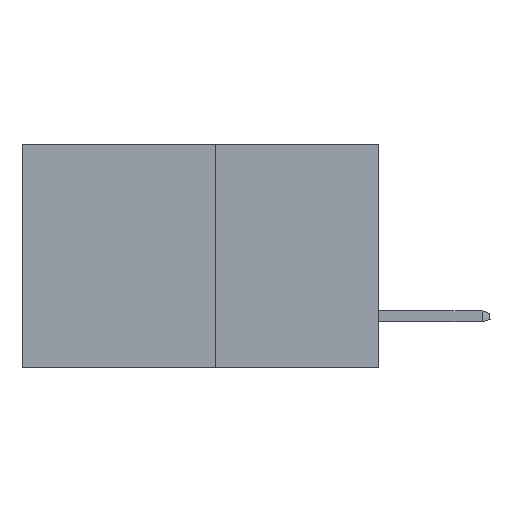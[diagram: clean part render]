
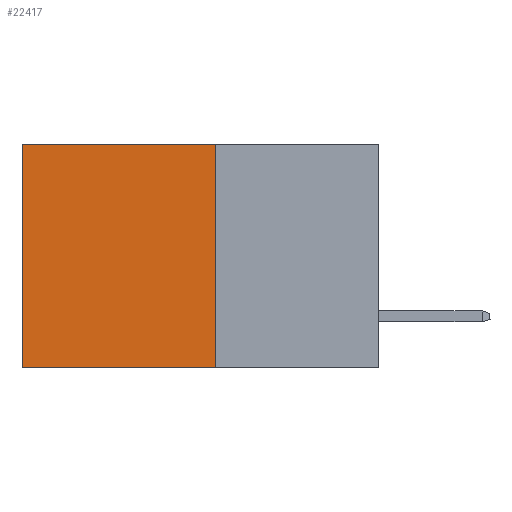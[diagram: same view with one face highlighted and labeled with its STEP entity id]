
A CAD part, left-side view. The second image highlights one B-rep face of the part: STEP entity #22417.
In plain terms, the highlighted planar face has unit normal (-1, 0, 0).
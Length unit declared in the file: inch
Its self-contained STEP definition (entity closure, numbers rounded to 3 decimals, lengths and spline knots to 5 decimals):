
#172 = VECTOR ( 'NONE', #13399, 39.37008 ) ;
#201 = LINE ( 'NONE', #4237, #14209 ) ;
#936 = VERTEX_POINT ( 'NONE', #5504 ) ;
#1294 = VERTEX_POINT ( 'NONE', #3661 ) ;
#1597 = DIRECTION ( 'NONE',  ( 1., 0., 0. ) ) ;
#2224 = ORIENTED_EDGE ( 'NONE', *, *, #5693, .F. ) ;
#2579 = EDGE_CURVE ( 'NONE', #5915, #1294, #22020, .T. ) ;
#2781 = AXIS2_PLACEMENT_3D ( 'NONE', #12547, #1597, #14374 ) ;
#3661 = CARTESIAN_POINT ( 'NONE',  ( 0.277, 0.27, -0.37 ) ) ;
#4237 = CARTESIAN_POINT ( 'NONE',  ( 0.277, 0.27, 0. ) ) ;
#5065 = EDGE_LOOP ( 'NONE', ( #9337, #2224, #10559, #20554 ) ) ;
#5504 = CARTESIAN_POINT ( 'NONE',  ( 0.277, 0.59, -0.37 ) ) ;
#5693 = EDGE_CURVE ( 'NONE', #1294, #936, #20147, .T. ) ;
#5915 = VERTEX_POINT ( 'NONE', #8877 ) ;
#8249 = CARTESIAN_POINT ( 'NONE',  ( 0.277, 0.59, -0.37 ) ) ;
#8877 = CARTESIAN_POINT ( 'NONE',  ( 0.277, 0.27, 0. ) ) ;
#9337 = ORIENTED_EDGE ( 'NONE', *, *, #19085, .T. ) ;
#9833 = CARTESIAN_POINT ( 'NONE',  ( 0.277, 0.27, -0.37 ) ) ;
#10106 = DIRECTION ( 'NONE',  ( 0., 0., -1. ) ) ;
#10559 = ORIENTED_EDGE ( 'NONE', *, *, #2579, .F. ) ;
#11546 = DIRECTION ( 'NONE',  ( 0., 1., 0. ) ) ;
#12547 = CARTESIAN_POINT ( 'NONE',  ( 0.277, 0.27, -0.37 ) ) ;
#13316 = FACE_OUTER_BOUND ( 'NONE', #5065, .T. ) ;
#13399 = DIRECTION ( 'NONE',  ( 0., 1., 0. ) ) ;
#13977 = VECTOR ( 'NONE', #10106, 39.37008 ) ;
#14209 = VECTOR ( 'NONE', #11546, 39.37008 ) ;
#14374 = DIRECTION ( 'NONE',  ( 0., 0., -1. ) ) ;
#14643 = CARTESIAN_POINT ( 'NONE',  ( 0.277, 0.59, 0. ) ) ;
#16384 = VERTEX_POINT ( 'NONE', #14643 ) ;
#16521 = VECTOR ( 'NONE', #19145, 39.37008 ) ;
#17156 = CARTESIAN_POINT ( 'NONE',  ( 0.277, 0.27, -0.37 ) ) ;
#18743 = LINE ( 'NONE', #8249, #13977 ) ;
#19085 = EDGE_CURVE ( 'NONE', #16384, #936, #18743, .T. ) ;
#19145 = DIRECTION ( 'NONE',  ( 0., 0., -1. ) ) ;
#20147 = LINE ( 'NONE', #9833, #172 ) ;
#20207 = EDGE_CURVE ( 'NONE', #5915, #16384, #201, .T. ) ;
#20554 = ORIENTED_EDGE ( 'NONE', *, *, #20207, .T. ) ;
#21656 = PLANE ( 'NONE',  #2781 ) ;
#22020 = LINE ( 'NONE', #17156, #16521 ) ;
#22417 = ADVANCED_FACE ( 'NONE', ( #13316 ), #21656, .F. ) ;
